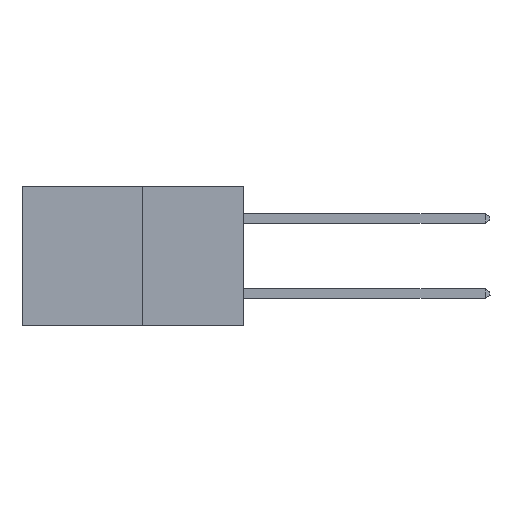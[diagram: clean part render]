
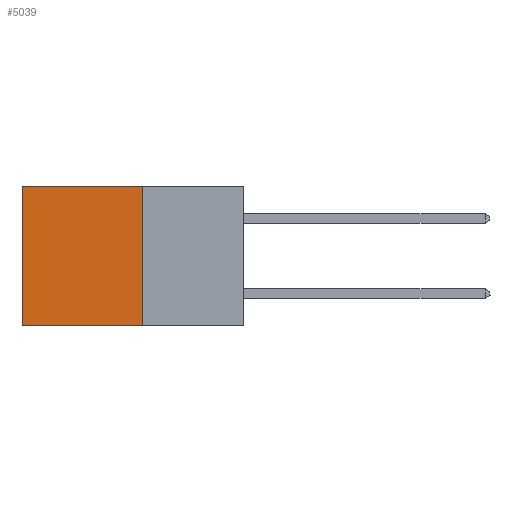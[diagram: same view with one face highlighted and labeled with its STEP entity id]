
A CAD part, left-side view. The second image highlights one B-rep face of the part: STEP entity #5039.
In plain terms, the highlighted planar face has unit normal (-1, 0, 0).
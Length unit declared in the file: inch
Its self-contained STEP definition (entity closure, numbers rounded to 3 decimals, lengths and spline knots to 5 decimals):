
#387 = EDGE_CURVE ( 'NONE', #11960, #17634, #4465, .T. ) ;
#1372 = EDGE_CURVE ( 'NONE', #16984, #11960, #12796, .T. ) ;
#2056 = EDGE_LOOP ( 'NONE', ( #10148, #15103, #27646, #15469 ) ) ;
#4465 = LINE ( 'NONE', #15263, #27558 ) ;
#5039 = ADVANCED_FACE ( 'NONE', ( #5183 ), #15833, .F. ) ;
#5183 = FACE_OUTER_BOUND ( 'NONE', #2056, .T. ) ;
#5263 = CARTESIAN_POINT ( 'NONE',  ( 0.277, 0.27, -0.37 ) ) ;
#6889 = VECTOR ( 'NONE', #23374, 39.37008 ) ;
#8289 = CARTESIAN_POINT ( 'NONE',  ( 0.277, 0.27, 0. ) ) ;
#8766 = VERTEX_POINT ( 'NONE', #13793 ) ;
#8982 = EDGE_CURVE ( 'NONE', #16984, #8766, #22322, .T. ) ;
#9053 = CARTESIAN_POINT ( 'NONE',  ( 0.277, 0.27, 0. ) ) ;
#10148 = ORIENTED_EDGE ( 'NONE', *, *, #24497, .T. ) ;
#11960 = VERTEX_POINT ( 'NONE', #22724 ) ;
#12796 = LINE ( 'NONE', #5263, #6889 ) ;
#13793 = CARTESIAN_POINT ( 'NONE',  ( 0.277, 0.59, 0. ) ) ;
#15064 = DIRECTION ( 'NONE',  ( 0., 1., 0. ) ) ;
#15103 = ORIENTED_EDGE ( 'NONE', *, *, #387, .F. ) ;
#15263 = CARTESIAN_POINT ( 'NONE',  ( 0.277, 0.27, -0.37 ) ) ;
#15469 = ORIENTED_EDGE ( 'NONE', *, *, #8982, .T. ) ;
#15539 = DIRECTION ( 'NONE',  ( 0., 0., -1. ) ) ;
#15747 = DIRECTION ( 'NONE',  ( 1., 0., 0. ) ) ;
#15833 = PLANE ( 'NONE',  #17044 ) ;
#16437 = VECTOR ( 'NONE', #15064, 39.37008 ) ;
#16468 = CARTESIAN_POINT ( 'NONE',  ( 0.277, 0.27, -0.37 ) ) ;
#16984 = VERTEX_POINT ( 'NONE', #9053 ) ;
#17044 = AXIS2_PLACEMENT_3D ( 'NONE', #16468, #15747, #15539 ) ;
#17589 = DIRECTION ( 'NONE',  ( 0., 1., 0. ) ) ;
#17634 = VERTEX_POINT ( 'NONE', #26888 ) ;
#22322 = LINE ( 'NONE', #8289, #16437 ) ;
#22724 = CARTESIAN_POINT ( 'NONE',  ( 0.277, 0.27, -0.37 ) ) ;
#23374 = DIRECTION ( 'NONE',  ( 0., 0., -1. ) ) ;
#23695 = CARTESIAN_POINT ( 'NONE',  ( 0.277, 0.59, -0.37 ) ) ;
#24497 = EDGE_CURVE ( 'NONE', #8766, #17634, #26046, .T. ) ;
#25382 = VECTOR ( 'NONE', #25914, 39.37008 ) ;
#25914 = DIRECTION ( 'NONE',  ( 0., 0., -1. ) ) ;
#26046 = LINE ( 'NONE', #23695, #25382 ) ;
#26888 = CARTESIAN_POINT ( 'NONE',  ( 0.277, 0.59, -0.37 ) ) ;
#27558 = VECTOR ( 'NONE', #17589, 39.37008 ) ;
#27646 = ORIENTED_EDGE ( 'NONE', *, *, #1372, .F. ) ;
